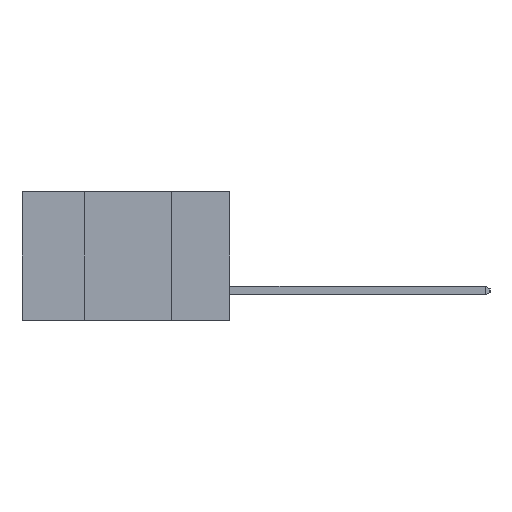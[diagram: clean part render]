
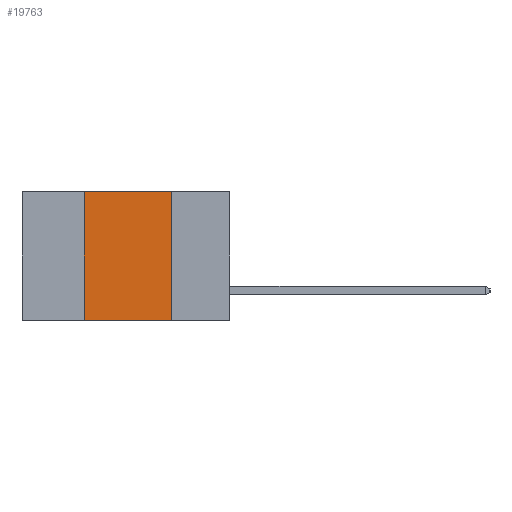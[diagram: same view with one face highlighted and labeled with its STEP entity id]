
A CAD part, left-side view. The second image highlights one B-rep face of the part: STEP entity #19763.
In plain terms, the highlighted planar face has unit normal (-1, 0, 0).
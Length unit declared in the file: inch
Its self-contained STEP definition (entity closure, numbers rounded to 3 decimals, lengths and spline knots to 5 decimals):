
#1014 = EDGE_CURVE ( 'NONE', #12193, #18029, #20527, .T. ) ;
#1362 = ORIENTED_EDGE ( 'NONE', *, *, #20336, .F. ) ;
#1591 = ORIENTED_EDGE ( 'NONE', *, *, #1014, .F. ) ;
#2069 = AXIS2_PLACEMENT_3D ( 'NONE', #10719, #4711, #18757 ) ;
#2677 = PLANE ( 'NONE',  #2069 ) ;
#2998 = LINE ( 'NONE', #17439, #17766 ) ;
#3385 = DIRECTION ( 'NONE',  ( 0., 0., -1. ) ) ;
#4711 = DIRECTION ( 'NONE',  ( 1., 0., 0. ) ) ;
#5137 = CARTESIAN_POINT ( 'NONE',  ( 0., 0.42, 0. ) ) ;
#6216 = CARTESIAN_POINT ( 'NONE',  ( 0., 0.17, -0.37 ) ) ;
#6876 = ORIENTED_EDGE ( 'NONE', *, *, #14975, .F. ) ;
#7220 = VERTEX_POINT ( 'NONE', #6216 ) ;
#7982 = DIRECTION ( 'NONE',  ( 0., -1., 0. ) ) ;
#8684 = FACE_OUTER_BOUND ( 'NONE', #22010, .T. ) ;
#9900 = VECTOR ( 'NONE', #11050, 39.37008 ) ;
#10719 = CARTESIAN_POINT ( 'NONE',  ( 0., 0.6, 0. ) ) ;
#11050 = DIRECTION ( 'NONE',  ( 0., 0., 1. ) ) ;
#11292 = VERTEX_POINT ( 'NONE', #12981 ) ;
#11384 = CARTESIAN_POINT ( 'NONE',  ( 0., 0.42, -0.37 ) ) ;
#12193 = VERTEX_POINT ( 'NONE', #13986 ) ;
#12981 = CARTESIAN_POINT ( 'NONE',  ( 0., 0.17, 0. ) ) ;
#13007 = CARTESIAN_POINT ( 'NONE',  ( 0., 0.6, -0.37 ) ) ;
#13964 = ORIENTED_EDGE ( 'NONE', *, *, #21813, .T. ) ;
#13986 = CARTESIAN_POINT ( 'NONE',  ( 0., 0.42, -0.37 ) ) ;
#14294 = VECTOR ( 'NONE', #7982, 39.37008 ) ;
#14975 = EDGE_CURVE ( 'NONE', #11292, #7220, #2998, .T. ) ;
#15114 = VECTOR ( 'NONE', #16936, 39.37008 ) ;
#16936 = DIRECTION ( 'NONE',  ( 0., -1., 0. ) ) ;
#17439 = CARTESIAN_POINT ( 'NONE',  ( 0., 0.17, -0.37 ) ) ;
#17766 = VECTOR ( 'NONE', #3385, 39.37008 ) ;
#18029 = VERTEX_POINT ( 'NONE', #5137 ) ;
#18757 = DIRECTION ( 'NONE',  ( 0., 0., -1. ) ) ;
#19597 = LINE ( 'NONE', #20055, #14294 ) ;
#19763 = ADVANCED_FACE ( 'NONE', ( #8684 ), #2677, .F. ) ;
#20055 = CARTESIAN_POINT ( 'NONE',  ( 0., 0.6, 0. ) ) ;
#20336 = EDGE_CURVE ( 'NONE', #18029, #11292, #19597, .T. ) ;
#20430 = LINE ( 'NONE', #13007, #15114 ) ;
#20527 = LINE ( 'NONE', #11384, #9900 ) ;
#21813 = EDGE_CURVE ( 'NONE', #12193, #7220, #20430, .T. ) ;
#22010 = EDGE_LOOP ( 'NONE', ( #6876, #1362, #1591, #13964 ) ) ;
